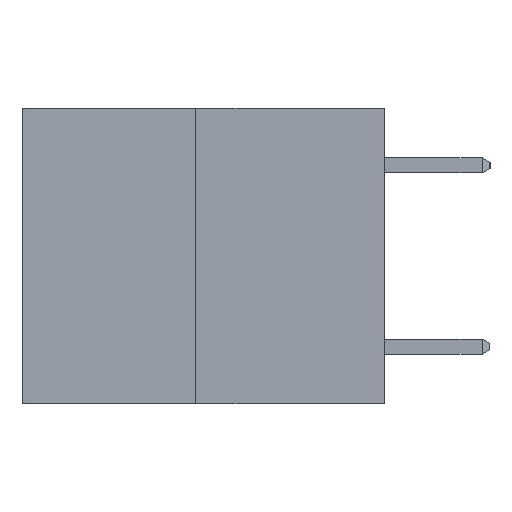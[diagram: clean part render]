
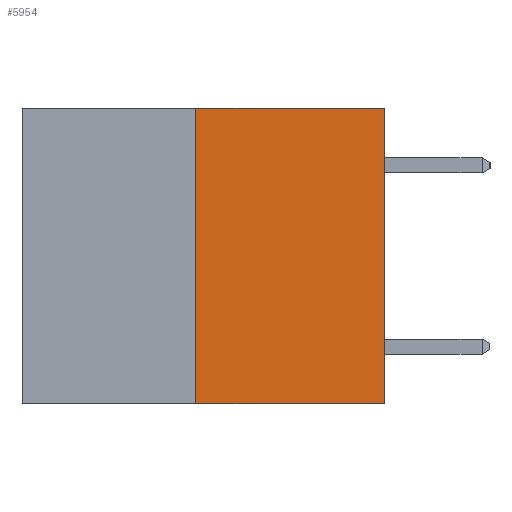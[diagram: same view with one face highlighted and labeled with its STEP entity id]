
A CAD part, left-side view. The second image highlights one B-rep face of the part: STEP entity #5954.
In plain terms, the highlighted planar face has unit normal (-1, 0, 0).
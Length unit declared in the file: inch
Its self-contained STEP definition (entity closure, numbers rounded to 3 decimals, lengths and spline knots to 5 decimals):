
#7 = CARTESIAN_POINT ( 'NONE',  ( 0., 0.312, -0.49 ) ) ;
#29 = DIRECTION ( 'NONE',  ( 0., -1., 0. ) ) ;
#72 = CARTESIAN_POINT ( 'NONE',  ( 0., 0., 0. ) ) ;
#262 = EDGE_CURVE ( 'NONE', #354, #3545, #8772, .T. ) ;
#300 = LINE ( 'NONE', #6650, #1183 ) ;
#346 = CARTESIAN_POINT ( 'NONE',  ( 0., 0.312, -0.49 ) ) ;
#354 = VERTEX_POINT ( 'NONE', #9222 ) ;
#1043 = LINE ( 'NONE', #346, #6724 ) ;
#1183 = VECTOR ( 'NONE', #5709, 39.37008 ) ;
#1294 = VECTOR ( 'NONE', #1738, 39.37008 ) ;
#1496 = VERTEX_POINT ( 'NONE', #7 ) ;
#1738 = DIRECTION ( 'NONE',  ( 0., 0., 1. ) ) ;
#3545 = VERTEX_POINT ( 'NONE', #5265 ) ;
#4535 = DIRECTION ( 'NONE',  ( 0., 0., 1. ) ) ;
#4960 = CARTESIAN_POINT ( 'NONE',  ( 0., 0.6, 0. ) ) ;
#5162 = VERTEX_POINT ( 'NONE', #6589 ) ;
#5265 = CARTESIAN_POINT ( 'NONE',  ( 0., 0., 0. ) ) ;
#5586 = CARTESIAN_POINT ( 'NONE',  ( 0., 0.6, 0. ) ) ;
#5648 = DIRECTION ( 'NONE',  ( 0., 0., -1. ) ) ;
#5709 = DIRECTION ( 'NONE',  ( 0., -1., 0. ) ) ;
#5806 = ORIENTED_EDGE ( 'NONE', *, *, #10632, .F. ) ;
#5954 = ADVANCED_FACE ( 'NONE', ( #10648 ), #10588, .F. ) ;
#6437 = AXIS2_PLACEMENT_3D ( 'NONE', #5586, #10672, #5648 ) ;
#6589 = CARTESIAN_POINT ( 'NONE',  ( 0., 0.312, 0. ) ) ;
#6650 = CARTESIAN_POINT ( 'NONE',  ( 0., 0.6, -0.49 ) ) ;
#6708 = LINE ( 'NONE', #4960, #7229 ) ;
#6724 = VECTOR ( 'NONE', #4535, 39.37008 ) ;
#6824 = ORIENTED_EDGE ( 'NONE', *, *, #7668, .T. ) ;
#7229 = VECTOR ( 'NONE', #29, 39.37008 ) ;
#7579 = EDGE_LOOP ( 'NONE', ( #9448, #6824, #7887, #5806 ) ) ;
#7668 = EDGE_CURVE ( 'NONE', #1496, #354, #300, .T. ) ;
#7887 = ORIENTED_EDGE ( 'NONE', *, *, #262, .T. ) ;
#8772 = LINE ( 'NONE', #72, #1294 ) ;
#9222 = CARTESIAN_POINT ( 'NONE',  ( 0., 0., -0.49 ) ) ;
#9448 = ORIENTED_EDGE ( 'NONE', *, *, #10274, .F. ) ;
#10274 = EDGE_CURVE ( 'NONE', #1496, #5162, #1043, .T. ) ;
#10588 = PLANE ( 'NONE',  #6437 ) ;
#10632 = EDGE_CURVE ( 'NONE', #5162, #3545, #6708, .T. ) ;
#10648 = FACE_OUTER_BOUND ( 'NONE', #7579, .T. ) ;
#10672 = DIRECTION ( 'NONE',  ( 1., 0., 0. ) ) ;
